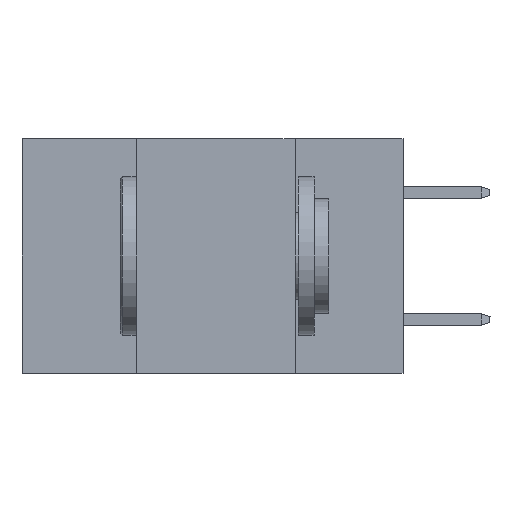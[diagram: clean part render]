
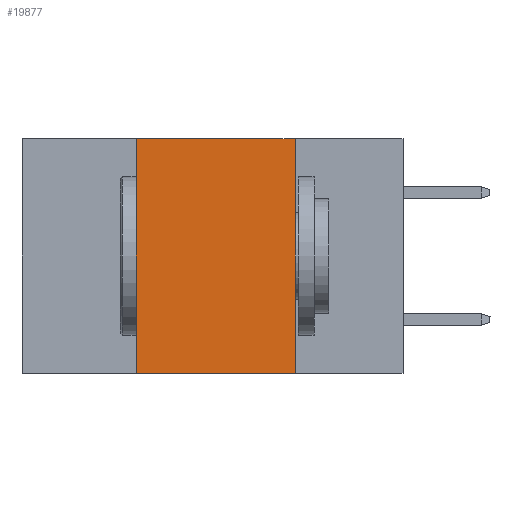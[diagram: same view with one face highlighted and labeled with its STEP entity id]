
A CAD part, left-side view. The second image highlights one B-rep face of the part: STEP entity #19877.
In plain terms, the highlighted planar face has unit normal (-1, 0, 0).
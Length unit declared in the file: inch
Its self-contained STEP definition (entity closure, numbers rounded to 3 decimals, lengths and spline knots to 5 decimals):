
#500 = CARTESIAN_POINT ( 'NONE',  ( 0., 0.17, 0. ) ) ;
#856 = EDGE_CURVE ( 'NONE', #1736, #6038, #16563, .T. ) ;
#1705 = VECTOR ( 'NONE', #20731, 39.37008 ) ;
#1736 = VERTEX_POINT ( 'NONE', #20105 ) ;
#2470 = DIRECTION ( 'NONE',  ( 0., 0., 1. ) ) ;
#2699 = EDGE_CURVE ( 'NONE', #12630, #1736, #5634, .T. ) ;
#3861 = DIRECTION ( 'NONE',  ( 0., 0., -1. ) ) ;
#4206 = DIRECTION ( 'NONE',  ( 0., 0., -1. ) ) ;
#5227 = VECTOR ( 'NONE', #3861, 39.37008 ) ;
#5456 = CARTESIAN_POINT ( 'NONE',  ( 0., 0.17, 0. ) ) ;
#5634 = LINE ( 'NONE', #16702, #12314 ) ;
#6038 = VERTEX_POINT ( 'NONE', #500 ) ;
#7179 = CARTESIAN_POINT ( 'NONE',  ( 0., 0.6, 0. ) ) ;
#7203 = ORIENTED_EDGE ( 'NONE', *, *, #19062, .F. ) ;
#7569 = EDGE_CURVE ( 'NONE', #12630, #12379, #8065, .T. ) ;
#7775 = CARTESIAN_POINT ( 'NONE',  ( 0., 0.17, -0.37 ) ) ;
#7845 = ORIENTED_EDGE ( 'NONE', *, *, #7569, .T. ) ;
#8065 = LINE ( 'NONE', #19036, #1705 ) ;
#8924 = PLANE ( 'NONE',  #20061 ) ;
#9328 = ORIENTED_EDGE ( 'NONE', *, *, #2699, .F. ) ;
#10602 = DIRECTION ( 'NONE',  ( 1., 0., 0. ) ) ;
#10970 = VECTOR ( 'NONE', #19835, 39.37008 ) ;
#11989 = FACE_OUTER_BOUND ( 'NONE', #18078, .T. ) ;
#12181 = CARTESIAN_POINT ( 'NONE',  ( 0., 0.6, 0. ) ) ;
#12314 = VECTOR ( 'NONE', #2470, 39.37008 ) ;
#12379 = VERTEX_POINT ( 'NONE', #7775 ) ;
#12630 = VERTEX_POINT ( 'NONE', #17032 ) ;
#15506 = ORIENTED_EDGE ( 'NONE', *, *, #856, .F. ) ;
#16563 = LINE ( 'NONE', #7179, #10970 ) ;
#16702 = CARTESIAN_POINT ( 'NONE',  ( 0., 0.42, 0. ) ) ;
#17032 = CARTESIAN_POINT ( 'NONE',  ( 0., 0.42, -0.37 ) ) ;
#18078 = EDGE_LOOP ( 'NONE', ( #7203, #15506, #9328, #7845 ) ) ;
#19036 = CARTESIAN_POINT ( 'NONE',  ( 0., 0.6, -0.37 ) ) ;
#19062 = EDGE_CURVE ( 'NONE', #6038, #12379, #19902, .T. ) ;
#19835 = DIRECTION ( 'NONE',  ( 0., -1., 0. ) ) ;
#19877 = ADVANCED_FACE ( 'NONE', ( #11989 ), #8924, .F. ) ;
#19902 = LINE ( 'NONE', #5456, #5227 ) ;
#20061 = AXIS2_PLACEMENT_3D ( 'NONE', #12181, #10602, #4206 ) ;
#20105 = CARTESIAN_POINT ( 'NONE',  ( 0., 0.42, 0. ) ) ;
#20731 = DIRECTION ( 'NONE',  ( 0., -1., 0. ) ) ;
